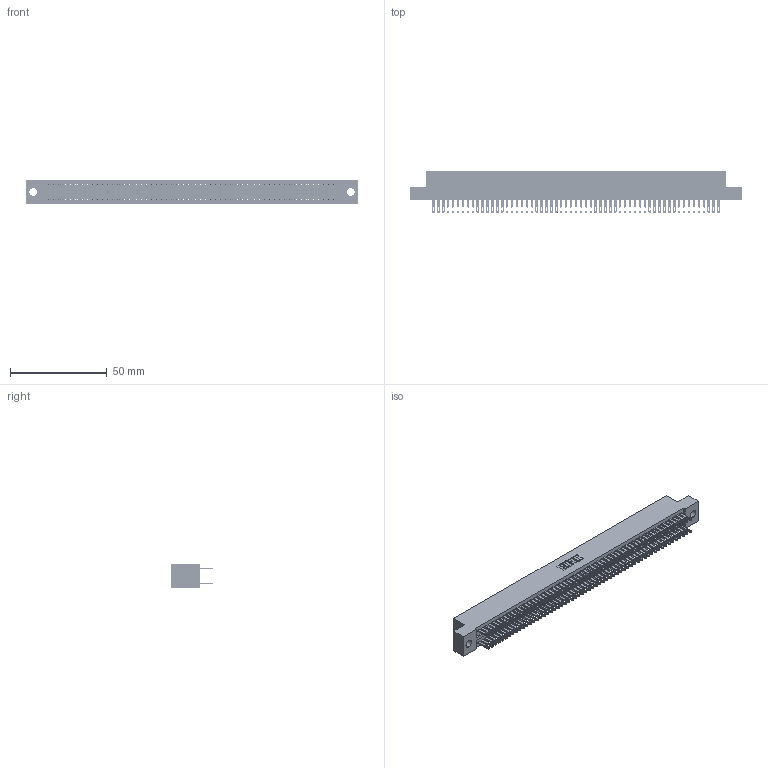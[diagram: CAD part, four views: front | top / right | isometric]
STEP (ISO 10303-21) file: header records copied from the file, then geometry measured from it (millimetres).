
FILE_DESCRIPTION (( 'STEP AP203' ), '1' );
FILE_NAME ('325-118-500-209.STEP', '2020-02-25T08:27:59', ( '' ), ( '' ), 'SwSTEP 2.0', 'SolidWorks 2016', '' );
FILE_SCHEMA (( 'CONFIG_CONTROL_DESIGN' ));
Length unit declared in the file: inch
Products named in the file (3): 325-292-001_325-293-100; 325-118-500-209; 325 Part_.160 TH
Assembly tree (119 placements, depth 2):
  325-118-500-209
    325 Part_.160 TH
    325-292-001_325-293-100  x118
Bounding box: 171.58 x 21.84 x 12.45 mm (x, y, z)
Volume: 22432.2 mm3; surface area: 28708.6 mm2
Topology: 119 solids, 119 shells, 5778 faces, 17657 edges, 11770 vertices
Faces by surface type: plane 3610, cylinder 2168
Entity records: 35691 total; most frequent: CARTESIAN_POINT 5894, ORIENTED_EDGE 5830, DIRECTION 5007, EDGE_CURVE 2915, VECTOR 2783, LINE 2783, VERTEX_POINT 1942, AXIS2_PLACEMENT_3D 1112
